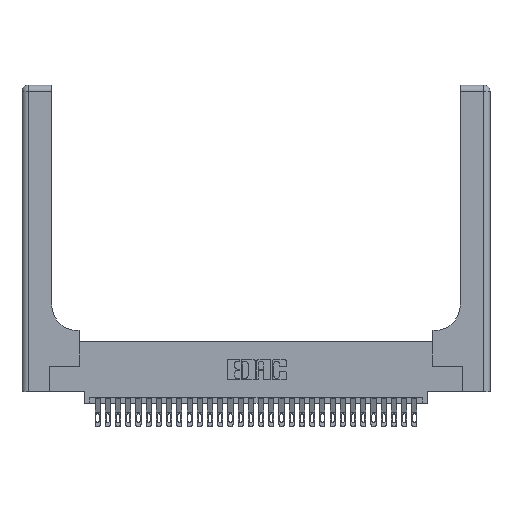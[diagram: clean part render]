
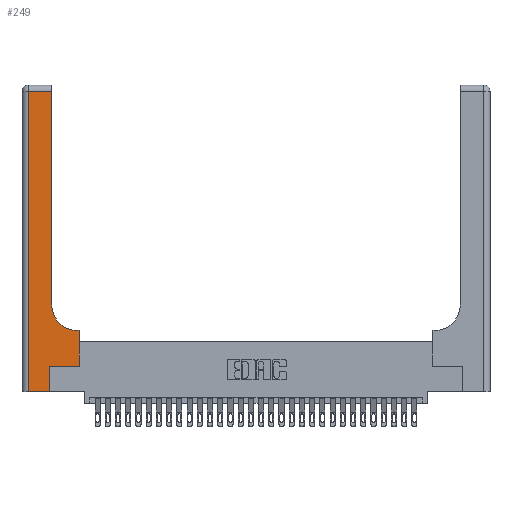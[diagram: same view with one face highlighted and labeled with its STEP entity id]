
A CAD part, top view. The second image highlights one B-rep face of the part: STEP entity #249.
In plain terms, the highlighted planar face has unit normal (0, 0, 1).
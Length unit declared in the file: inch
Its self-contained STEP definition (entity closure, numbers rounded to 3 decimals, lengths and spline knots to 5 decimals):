
#249 = ADVANCED_FACE ( 'NONE', ( #20096 ), #31811, .F. ) ;
#1038 = DIRECTION ( 'NONE',  ( -1., 0., 0. ) ) ;
#1677 = CARTESIAN_POINT ( 'NONE',  ( 0.5585, 0.6, 0.37 ) ) ;
#1991 = EDGE_CURVE ( 'NONE', #23159, #18670, #30877, .T. ) ;
#3000 = DIRECTION ( 'NONE',  ( 0., 1., 0. ) ) ;
#3624 = CIRCLE ( 'NONE', #24687, 0.25 ) ;
#3764 = VERTEX_POINT ( 'NONE', #30581 ) ;
#5580 = DIRECTION ( 'NONE',  ( 0., 0., -1. ) ) ;
#5671 = LINE ( 'NONE', #13300, #24715 ) ;
#6126 = EDGE_CURVE ( 'NONE', #26396, #3764, #15544, .T. ) ;
#6331 = CARTESIAN_POINT ( 'NONE',  ( 0.5585, 0.25, 0.37 ) ) ;
#7092 = CARTESIAN_POINT ( 'NONE',  ( 0.269, 0., 0.37 ) ) ;
#7944 = CARTESIAN_POINT ( 'NONE',  ( 0.2915, 0.85, 0.37 ) ) ;
#7976 = DIRECTION ( 'NONE',  ( 0., -1., 0. ) ) ;
#8254 = CARTESIAN_POINT ( 'NONE',  ( 0.2915, 3., 0.37 ) ) ;
#8548 = ORIENTED_EDGE ( 'NONE', *, *, #10672, .T. ) ;
#8585 = EDGE_CURVE ( 'NONE', #14209, #23159, #17365, .T. ) ;
#8619 = ORIENTED_EDGE ( 'NONE', *, *, #25684, .T. ) ;
#8657 = ORIENTED_EDGE ( 'NONE', *, *, #12171, .T. ) ;
#9186 = VECTOR ( 'NONE', #10453, 39.37008 ) ;
#9360 = EDGE_CURVE ( 'NONE', #18090, #14209, #10692, .T. ) ;
#10453 = DIRECTION ( 'NONE',  ( 1., 0., 0. ) ) ;
#10549 = DIRECTION ( 'NONE',  ( 1., 0., 0. ) ) ;
#10672 = EDGE_CURVE ( 'NONE', #31274, #18090, #3624, .T. ) ;
#10692 = LINE ( 'NONE', #8254, #23112 ) ;
#11135 = VECTOR ( 'NONE', #23696, 39.37008 ) ;
#12171 = EDGE_CURVE ( 'NONE', #3764, #20339, #15817, .T. ) ;
#12763 = CARTESIAN_POINT ( 'NONE',  ( 0.06, 3., 0.37 ) ) ;
#13300 = CARTESIAN_POINT ( 'NONE',  ( 0.2915, 0.6, 0.37 ) ) ;
#13597 = VECTOR ( 'NONE', #24752, 39.37008 ) ;
#13879 = LINE ( 'NONE', #6331, #11135 ) ;
#14209 = VERTEX_POINT ( 'NONE', #23296 ) ;
#15065 = ORIENTED_EDGE ( 'NONE', *, *, #16874, .T. ) ;
#15544 = LINE ( 'NONE', #7092, #15923 ) ;
#15682 = ORIENTED_EDGE ( 'NONE', *, *, #9360, .T. ) ;
#15817 = LINE ( 'NONE', #27281, #9186 ) ;
#15923 = VECTOR ( 'NONE', #24471, 39.37008 ) ;
#16874 = EDGE_CURVE ( 'NONE', #18670, #26396, #26804, .T. ) ;
#17365 = LINE ( 'NONE', #18619, #28985 ) ;
#18090 = VERTEX_POINT ( 'NONE', #7944 ) ;
#18619 = CARTESIAN_POINT ( 'NONE',  ( 0., 2.94, 0.37 ) ) ;
#18670 = VERTEX_POINT ( 'NONE', #29934 ) ;
#20013 = CARTESIAN_POINT ( 'NONE',  ( 0.06, 2.94, 0.37 ) ) ;
#20096 = FACE_OUTER_BOUND ( 'NONE', #27587, .T. ) ;
#20339 = VERTEX_POINT ( 'NONE', #27150 ) ;
#21143 = EDGE_CURVE ( 'NONE', #28693, #31274, #5671, .T. ) ;
#22230 = CARTESIAN_POINT ( 'NONE',  ( 0., 0., 0.37 ) ) ;
#22768 = DIRECTION ( 'NONE',  ( -1., 0., 0. ) ) ;
#22929 = CARTESIAN_POINT ( 'NONE',  ( 0.5415, 0.85, 0.37 ) ) ;
#22947 = ORIENTED_EDGE ( 'NONE', *, *, #1991, .T. ) ;
#23112 = VECTOR ( 'NONE', #3000, 39.37008 ) ;
#23159 = VERTEX_POINT ( 'NONE', #20013 ) ;
#23296 = CARTESIAN_POINT ( 'NONE',  ( 0.2915, 2.94, 0.37 ) ) ;
#23445 = ORIENTED_EDGE ( 'NONE', *, *, #21143, .T. ) ;
#23696 = DIRECTION ( 'NONE',  ( 0., 1., 0. ) ) ;
#24296 = ORIENTED_EDGE ( 'NONE', *, *, #6126, .T. ) ;
#24471 = DIRECTION ( 'NONE',  ( 0., 1., 0. ) ) ;
#24687 = AXIS2_PLACEMENT_3D ( 'NONE', #22929, #5580, #10549 ) ;
#24715 = VECTOR ( 'NONE', #22768, 39.37008 ) ;
#24752 = DIRECTION ( 'NONE',  ( 1., 0., 0. ) ) ;
#25460 = VECTOR ( 'NONE', #7976, 39.37008 ) ;
#25684 = EDGE_CURVE ( 'NONE', #20339, #28693, #13879, .T. ) ;
#26396 = VERTEX_POINT ( 'NONE', #29948 ) ;
#26804 = LINE ( 'NONE', #22230, #13597 ) ;
#26941 = DIRECTION ( 'NONE',  ( 0., 0., -1. ) ) ;
#27150 = CARTESIAN_POINT ( 'NONE',  ( 0.5585, 0.25, 0.37 ) ) ;
#27281 = CARTESIAN_POINT ( 'NONE',  ( 0.269, 0.25, 0.37 ) ) ;
#27537 = ORIENTED_EDGE ( 'NONE', *, *, #8585, .T. ) ;
#27587 = EDGE_LOOP ( 'NONE', ( #15682, #27537, #22947, #15065, #24296, #8657, #8619, #23445, #8548 ) ) ;
#28693 = VERTEX_POINT ( 'NONE', #1677 ) ;
#28985 = VECTOR ( 'NONE', #1038, 39.37008 ) ;
#29030 = CARTESIAN_POINT ( 'NONE',  ( 0.5415, 0.6, 0.37 ) ) ;
#29540 = CARTESIAN_POINT ( 'NONE',  ( 0., 3., 0.37 ) ) ;
#29648 = DIRECTION ( 'NONE',  ( -1., 0., 0. ) ) ;
#29934 = CARTESIAN_POINT ( 'NONE',  ( 0.06, 0., 0.37 ) ) ;
#29948 = CARTESIAN_POINT ( 'NONE',  ( 0.269, 0., 0.37 ) ) ;
#30581 = CARTESIAN_POINT ( 'NONE',  ( 0.269, 0.25, 0.37 ) ) ;
#30877 = LINE ( 'NONE', #12763, #25460 ) ;
#31135 = AXIS2_PLACEMENT_3D ( 'NONE', #29540, #26941, #29648 ) ;
#31274 = VERTEX_POINT ( 'NONE', #29030 ) ;
#31811 = PLANE ( 'NONE',  #31135 ) ;
